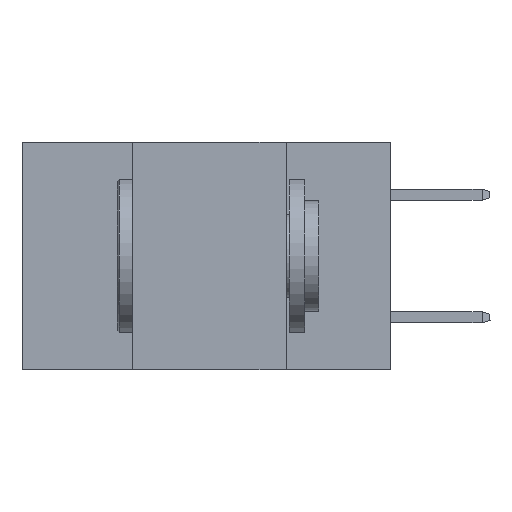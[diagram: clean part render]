
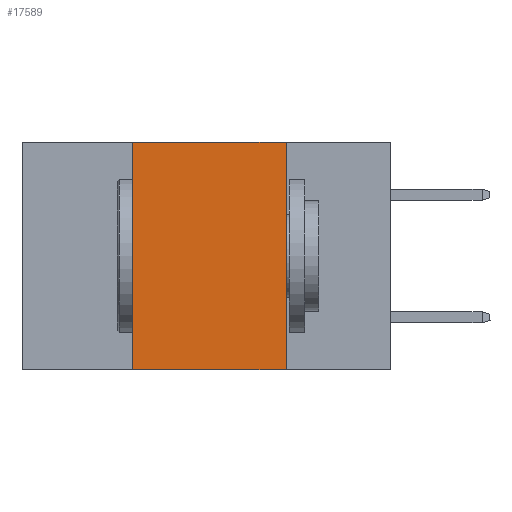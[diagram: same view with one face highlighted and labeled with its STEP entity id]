
A CAD part, left-side view. The second image highlights one B-rep face of the part: STEP entity #17589.
In plain terms, the highlighted planar face has unit normal (-1, 0, 0).
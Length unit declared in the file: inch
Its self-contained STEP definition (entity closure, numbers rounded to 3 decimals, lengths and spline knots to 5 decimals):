
#295 = FACE_OUTER_BOUND ( 'NONE', #5635, .T. ) ;
#379 = ORIENTED_EDGE ( 'NONE', *, *, #7835, .T. ) ;
#600 = ORIENTED_EDGE ( 'NONE', *, *, #15640, .F. ) ;
#681 = LINE ( 'NONE', #8050, #19443 ) ;
#842 = CARTESIAN_POINT ( 'NONE',  ( 0., 0.6, 0. ) ) ;
#1890 = VERTEX_POINT ( 'NONE', #5284 ) ;
#2008 = CARTESIAN_POINT ( 'NONE',  ( 0., 0.6, 0. ) ) ;
#2642 = PLANE ( 'NONE',  #6934 ) ;
#3187 = CARTESIAN_POINT ( 'NONE',  ( 0., 0.42, 0. ) ) ;
#3630 = CARTESIAN_POINT ( 'NONE',  ( 0., 0.17, 0. ) ) ;
#4564 = DIRECTION ( 'NONE',  ( 0., -1., 0. ) ) ;
#4846 = LINE ( 'NONE', #2008, #18272 ) ;
#5284 = CARTESIAN_POINT ( 'NONE',  ( 0., 0.17, -0.37 ) ) ;
#5376 = DIRECTION ( 'NONE',  ( 0., 0., -1. ) ) ;
#5635 = EDGE_LOOP ( 'NONE', ( #18091, #13409, #600, #379 ) ) ;
#5764 = VERTEX_POINT ( 'NONE', #14245 ) ;
#5808 = CARTESIAN_POINT ( 'NONE',  ( 0., 0.17, 0. ) ) ;
#6199 = DIRECTION ( 'NONE',  ( 0., 0., -1. ) ) ;
#6934 = AXIS2_PLACEMENT_3D ( 'NONE', #842, #16672, #6199 ) ;
#7483 = LINE ( 'NONE', #3187, #20904 ) ;
#7835 = EDGE_CURVE ( 'NONE', #10532, #1890, #681, .T. ) ;
#8050 = CARTESIAN_POINT ( 'NONE',  ( 0., 0.6, -0.37 ) ) ;
#8481 = CARTESIAN_POINT ( 'NONE',  ( 0., 0.42, -0.37 ) ) ;
#9409 = EDGE_CURVE ( 'NONE', #5764, #15272, #4846, .T. ) ;
#10532 = VERTEX_POINT ( 'NONE', #8481 ) ;
#11433 = EDGE_CURVE ( 'NONE', #15272, #1890, #12845, .T. ) ;
#12313 = VECTOR ( 'NONE', #5376, 39.37008 ) ;
#12845 = LINE ( 'NONE', #3630, #12313 ) ;
#13409 = ORIENTED_EDGE ( 'NONE', *, *, #9409, .F. ) ;
#14245 = CARTESIAN_POINT ( 'NONE',  ( 0., 0.42, 0. ) ) ;
#15272 = VERTEX_POINT ( 'NONE', #5808 ) ;
#15640 = EDGE_CURVE ( 'NONE', #10532, #5764, #7483, .T. ) ;
#16044 = DIRECTION ( 'NONE',  ( 0., -1., 0. ) ) ;
#16672 = DIRECTION ( 'NONE',  ( 1., 0., 0. ) ) ;
#17589 = ADVANCED_FACE ( 'NONE', ( #295 ), #2642, .F. ) ;
#18091 = ORIENTED_EDGE ( 'NONE', *, *, #11433, .F. ) ;
#18272 = VECTOR ( 'NONE', #16044, 39.37008 ) ;
#18939 = DIRECTION ( 'NONE',  ( 0., 0., 1. ) ) ;
#19443 = VECTOR ( 'NONE', #4564, 39.37008 ) ;
#20904 = VECTOR ( 'NONE', #18939, 39.37008 ) ;
